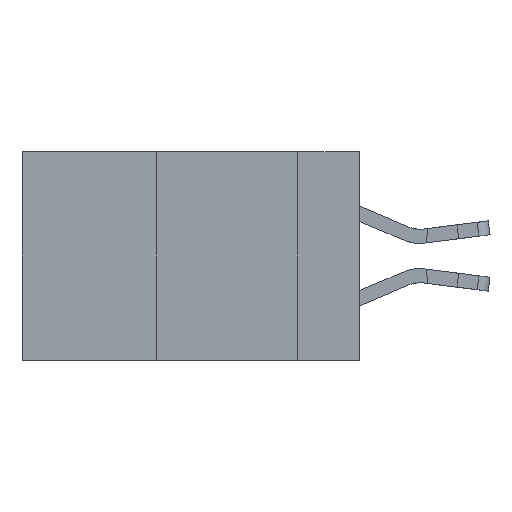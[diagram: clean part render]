
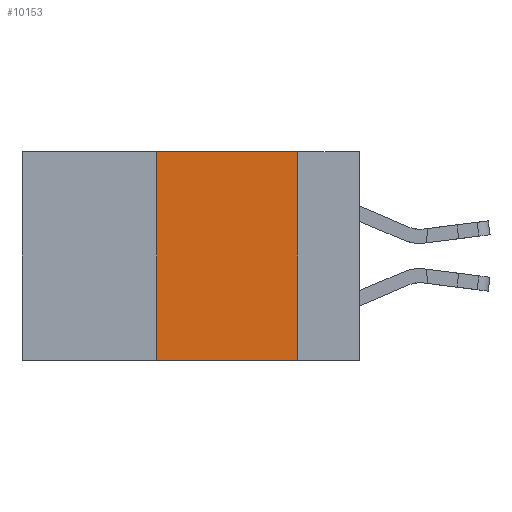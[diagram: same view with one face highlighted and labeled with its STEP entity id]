
A CAD part, left-side view. The second image highlights one B-rep face of the part: STEP entity #10153.
In plain terms, the highlighted planar face has unit normal (-1, 0, 0).
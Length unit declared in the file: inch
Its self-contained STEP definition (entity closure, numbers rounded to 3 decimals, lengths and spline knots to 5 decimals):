
#646 = VERTEX_POINT ( 'NONE', #15657 ) ;
#1019 = CARTESIAN_POINT ( 'NONE',  ( 0., 0.36, 0. ) ) ;
#1099 = ORIENTED_EDGE ( 'NONE', *, *, #10970, .F. ) ;
#2810 = CARTESIAN_POINT ( 'NONE',  ( 0., 0.36, -0.37 ) ) ;
#2910 = AXIS2_PLACEMENT_3D ( 'NONE', #17732, #8439, #12153 ) ;
#4007 = DIRECTION ( 'NONE',  ( 0., -1., 0. ) ) ;
#4097 = CARTESIAN_POINT ( 'NONE',  ( 0., 0.6, 0. ) ) ;
#4438 = ORIENTED_EDGE ( 'NONE', *, *, #6346, .F. ) ;
#4684 = VECTOR ( 'NONE', #15086, 39.37008 ) ;
#5050 = VERTEX_POINT ( 'NONE', #17143 ) ;
#5396 = CARTESIAN_POINT ( 'NONE',  ( 0., 0.6, -0.37 ) ) ;
#5452 = LINE ( 'NONE', #1019, #9194 ) ;
#5749 = EDGE_CURVE ( 'NONE', #19640, #646, #14043, .T. ) ;
#6243 = VECTOR ( 'NONE', #4007, 39.37008 ) ;
#6346 = EDGE_CURVE ( 'NONE', #19640, #5050, #5452, .T. ) ;
#8439 = DIRECTION ( 'NONE',  ( 1., 0., 0. ) ) ;
#9191 = VECTOR ( 'NONE', #18086, 39.37008 ) ;
#9194 = VECTOR ( 'NONE', #13815, 39.37008 ) ;
#10153 = ADVANCED_FACE ( 'NONE', ( #14277 ), #15675, .F. ) ;
#10945 = ORIENTED_EDGE ( 'NONE', *, *, #20861, .F. ) ;
#10970 = EDGE_CURVE ( 'NONE', #5050, #12329, #13966, .T. ) ;
#12153 = DIRECTION ( 'NONE',  ( 0., 0., -1. ) ) ;
#12329 = VERTEX_POINT ( 'NONE', #19519 ) ;
#12687 = LINE ( 'NONE', #20561, #4684 ) ;
#13235 = EDGE_LOOP ( 'NONE', ( #10945, #1099, #4438, #18753 ) ) ;
#13815 = DIRECTION ( 'NONE',  ( 0., 0., 1. ) ) ;
#13966 = LINE ( 'NONE', #4097, #6243 ) ;
#14043 = LINE ( 'NONE', #5396, #9191 ) ;
#14277 = FACE_OUTER_BOUND ( 'NONE', #13235, .T. ) ;
#15086 = DIRECTION ( 'NONE',  ( 0., 0., -1. ) ) ;
#15657 = CARTESIAN_POINT ( 'NONE',  ( 0., 0.11, -0.37 ) ) ;
#15675 = PLANE ( 'NONE',  #2910 ) ;
#17143 = CARTESIAN_POINT ( 'NONE',  ( 0., 0.36, 0. ) ) ;
#17732 = CARTESIAN_POINT ( 'NONE',  ( 0., 0.6, 0. ) ) ;
#18086 = DIRECTION ( 'NONE',  ( 0., -1., 0. ) ) ;
#18753 = ORIENTED_EDGE ( 'NONE', *, *, #5749, .T. ) ;
#19519 = CARTESIAN_POINT ( 'NONE',  ( 0., 0.11, 0. ) ) ;
#19640 = VERTEX_POINT ( 'NONE', #2810 ) ;
#20561 = CARTESIAN_POINT ( 'NONE',  ( 0., 0.11, 0. ) ) ;
#20861 = EDGE_CURVE ( 'NONE', #12329, #646, #12687, .T. ) ;
